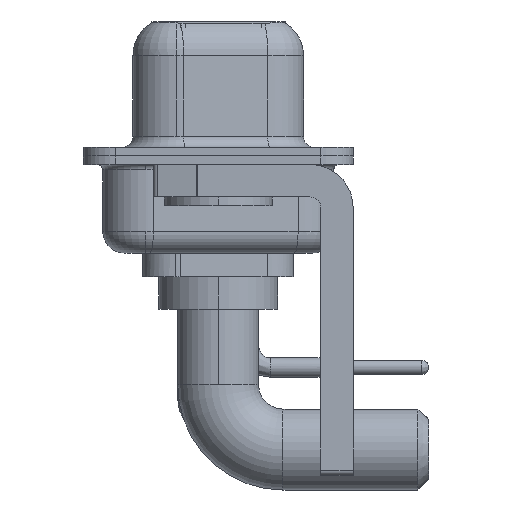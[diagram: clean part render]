
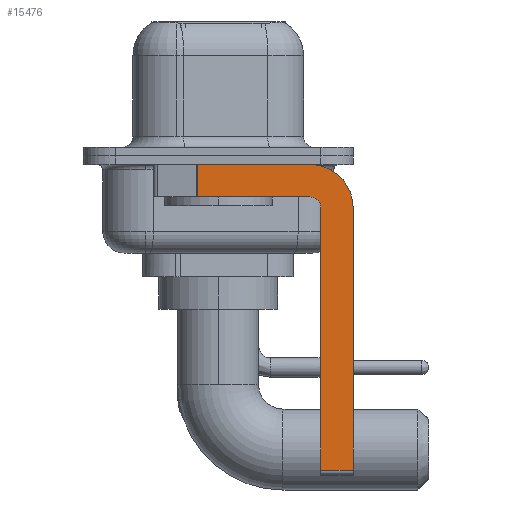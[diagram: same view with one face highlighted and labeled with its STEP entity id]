
A CAD part, left-side view. The second image highlights one B-rep face of the part: STEP entity #15476.
In plain terms, the highlighted planar face has unit normal (-1, 0, 0).
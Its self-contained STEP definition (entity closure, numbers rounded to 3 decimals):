
#264 = PLANE ( 'NONE',  #19410 ) ;
#449 = ORIENTED_EDGE ( 'NONE', *, *, #16894, .F. ) ;
#1013 = CARTESIAN_POINT ( 'NONE',  ( -2.9, -4.25, -1.9 ) ) ;
#1363 = VERTEX_POINT ( 'NONE', #2961 ) ;
#1411 = ORIENTED_EDGE ( 'NONE', *, *, #4448, .F. ) ;
#1781 = CARTESIAN_POINT ( 'NONE',  ( -2.9, 0.978, -1.9 ) ) ;
#2254 = ORIENTED_EDGE ( 'NONE', *, *, #6448, .F. ) ;
#2817 = CARTESIAN_POINT ( 'NONE',  ( -2.9, -6.25, -2.4 ) ) ;
#2961 = CARTESIAN_POINT ( 'NONE',  ( -2.9, -4.25, -1.9 ) ) ;
#3042 = VERTEX_POINT ( 'NONE', #8206 ) ;
#3604 = CARTESIAN_POINT ( 'NONE',  ( -2.9, -4.25, -2.4 ) ) ;
#3623 = DIRECTION ( 'NONE',  ( 0., 0., -1. ) ) ;
#4056 = DIRECTION ( 'NONE',  ( 1., 0., 0. ) ) ;
#4257 = CARTESIAN_POINT ( 'NONE',  ( -2.9, -4.25, -2.4 ) ) ;
#4448 = EDGE_CURVE ( 'NONE', #20336, #21342, #20787, .T. ) ;
#4487 = DIRECTION ( 'NONE',  ( 0., 0., -1. ) ) ;
#5126 = DIRECTION ( 'NONE',  ( -1., 0., 0. ) ) ;
#5162 = ORIENTED_EDGE ( 'NONE', *, *, #9067, .T. ) ;
#5437 = VECTOR ( 'NONE', #12216, 1000. ) ;
#5533 = AXIS2_PLACEMENT_3D ( 'NONE', #17251, #5126, #6832 ) ;
#6364 = VECTOR ( 'NONE', #10869, 1000. ) ;
#6448 = EDGE_CURVE ( 'NONE', #20627, #13278, #10751, .T. ) ;
#6832 = DIRECTION ( 'NONE',  ( 0., 0., 1. ) ) ;
#7201 = CARTESIAN_POINT ( 'NONE',  ( -2.9, 0.978, -1.9 ) ) ;
#7366 = CIRCLE ( 'NONE', #5533, 0.5 ) ;
#7496 = AXIS2_PLACEMENT_3D ( 'NONE', #4257, #15083, #4487 ) ;
#7500 = FACE_OUTER_BOUND ( 'NONE', #10106, .T. ) ;
#8206 = CARTESIAN_POINT ( 'NONE',  ( -2.9, -6.25, -14.55 ) ) ;
#8295 = VECTOR ( 'NONE', #21131, 1000. ) ;
#8331 = LINE ( 'NONE', #2817, #15760 ) ;
#8906 = LINE ( 'NONE', #1781, #22212 ) ;
#9003 = LINE ( 'NONE', #17568, #8295 ) ;
#9005 = ORIENTED_EDGE ( 'NONE', *, *, #12590, .T. ) ;
#9067 = EDGE_CURVE ( 'NONE', #20336, #17695, #8906, .T. ) ;
#9772 = ORIENTED_EDGE ( 'NONE', *, *, #15313, .F. ) ;
#10106 = EDGE_LOOP ( 'NONE', ( #1411, #5162, #9772, #11104, #2254, #9005, #449, #19071 ) ) ;
#10751 = LINE ( 'NONE', #14455, #6364 ) ;
#10869 = DIRECTION ( 'NONE',  ( 0., 0., 1. ) ) ;
#11104 = ORIENTED_EDGE ( 'NONE', *, *, #19597, .F. ) ;
#11230 = CARTESIAN_POINT ( 'NONE',  ( -2.9, -6.25, -2.4 ) ) ;
#11428 = EDGE_CURVE ( 'NONE', #21342, #11881, #17819, .T. ) ;
#11628 = CARTESIAN_POINT ( 'NONE',  ( -2.9, -4.75, -2.4 ) ) ;
#11881 = VERTEX_POINT ( 'NONE', #11230 ) ;
#12216 = DIRECTION ( 'NONE',  ( 0., -1., 0. ) ) ;
#12590 = EDGE_CURVE ( 'NONE', #20627, #3042, #9003, .T. ) ;
#13197 = DIRECTION ( 'NONE',  ( 0., 1., 0. ) ) ;
#13278 = VERTEX_POINT ( 'NONE', #11628 ) ;
#13283 = DIRECTION ( 'NONE',  ( 0., 0., -1. ) ) ;
#13803 = CARTESIAN_POINT ( 'NONE',  ( -2.9, 0.978, -0.4 ) ) ;
#14308 = DIRECTION ( 'NONE',  ( 0., 0., -1. ) ) ;
#14455 = CARTESIAN_POINT ( 'NONE',  ( -2.9, -4.75, -14.8 ) ) ;
#14933 = LINE ( 'NONE', #1013, #18664 ) ;
#15083 = DIRECTION ( 'NONE',  ( 1., 0., 0. ) ) ;
#15313 = EDGE_CURVE ( 'NONE', #1363, #17695, #14933, .T. ) ;
#15476 = ADVANCED_FACE ( 'NONE', ( #7500 ), #264, .F. ) ;
#15760 = VECTOR ( 'NONE', #13283, 1000. ) ;
#16894 = EDGE_CURVE ( 'NONE', #11881, #3042, #8331, .T. ) ;
#17251 = CARTESIAN_POINT ( 'NONE',  ( -2.9, -4.25, -2.4 ) ) ;
#17568 = CARTESIAN_POINT ( 'NONE',  ( -2.9, -4.25, -14.55 ) ) ;
#17695 = VERTEX_POINT ( 'NONE', #7201 ) ;
#17819 = CIRCLE ( 'NONE', #7496, 2. ) ;
#18619 = CARTESIAN_POINT ( 'NONE',  ( -2.9, -4.25, -0.4 ) ) ;
#18664 = VECTOR ( 'NONE', #13197, 1000. ) ;
#19071 = ORIENTED_EDGE ( 'NONE', *, *, #11428, .F. ) ;
#19410 = AXIS2_PLACEMENT_3D ( 'NONE', #3604, #4056, #14308 ) ;
#19597 = EDGE_CURVE ( 'NONE', #13278, #1363, #7366, .T. ) ;
#20336 = VERTEX_POINT ( 'NONE', #13803 ) ;
#20627 = VERTEX_POINT ( 'NONE', #21870 ) ;
#20787 = LINE ( 'NONE', #22525, #5437 ) ;
#21131 = DIRECTION ( 'NONE',  ( 0., -1., 0. ) ) ;
#21342 = VERTEX_POINT ( 'NONE', #18619 ) ;
#21870 = CARTESIAN_POINT ( 'NONE',  ( -2.9, -4.75, -14.55 ) ) ;
#22212 = VECTOR ( 'NONE', #3623, 1000. ) ;
#22525 = CARTESIAN_POINT ( 'NONE',  ( -2.9, 3., -0.4 ) ) ;
